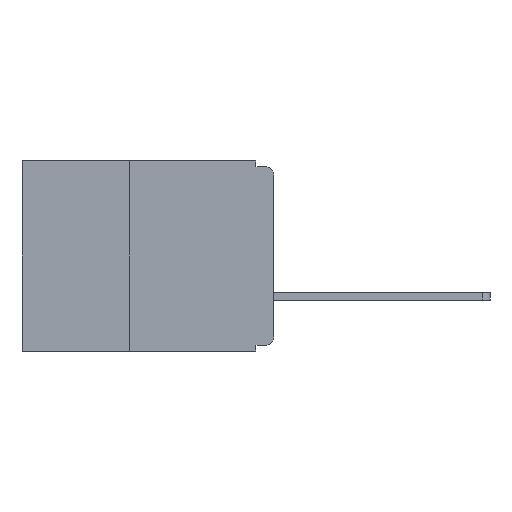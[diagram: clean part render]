
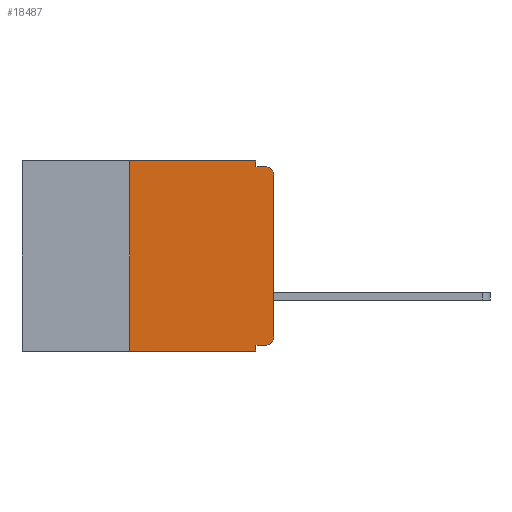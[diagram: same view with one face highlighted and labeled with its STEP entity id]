
A CAD part, left-side view. The second image highlights one B-rep face of the part: STEP entity #18487.
In plain terms, the highlighted planar face has unit normal (-1, 0, 0).
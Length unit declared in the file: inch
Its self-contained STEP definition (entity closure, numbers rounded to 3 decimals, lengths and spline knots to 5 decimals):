
#346 = LINE ( 'NONE', #22528, #4045 ) ;
#390 = ORIENTED_EDGE ( 'NONE', *, *, #810, .F. ) ;
#554 = CARTESIAN_POINT ( 'NONE',  ( 0., 0., -0.305 ) ) ;
#629 = ORIENTED_EDGE ( 'NONE', *, *, #4775, .T. ) ;
#810 = EDGE_CURVE ( 'NONE', #17981, #12182, #4354, .T. ) ;
#930 = DIRECTION ( 'NONE',  ( 0., 0., 1. ) ) ;
#1153 = PLANE ( 'NONE',  #10870 ) ;
#1577 = EDGE_CURVE ( 'NONE', #4454, #16784, #15068, .T. ) ;
#2307 = DIRECTION ( 'NONE',  ( -1., 0., 0. ) ) ;
#2333 = VECTOR ( 'NONE', #21687, 39.37008 ) ;
#2358 = DIRECTION ( 'NONE',  ( 0., 0., -1. ) ) ;
#2964 = DIRECTION ( 'NONE',  ( 0., 0., -1. ) ) ;
#4045 = VECTOR ( 'NONE', #930, 39.37008 ) ;
#4226 = LINE ( 'NONE', #22168, #21694 ) ;
#4227 = VECTOR ( 'NONE', #13757, 39.37008 ) ;
#4354 = LINE ( 'NONE', #13585, #18213 ) ;
#4454 = VERTEX_POINT ( 'NONE', #20474 ) ;
#4615 = VERTEX_POINT ( 'NONE', #11181 ) ;
#4775 = EDGE_CURVE ( 'NONE', #9815, #13558, #23043, .T. ) ;
#5423 = VERTEX_POINT ( 'NONE', #13109 ) ;
#5455 = VECTOR ( 'NONE', #10289, 39.37008 ) ;
#5767 = VECTOR ( 'NONE', #2358, 39.37008 ) ;
#5929 = EDGE_CURVE ( 'NONE', #4615, #17981, #7806, .T. ) ;
#6445 = FACE_OUTER_BOUND ( 'NONE', #19555, .T. ) ;
#7180 = CARTESIAN_POINT ( 'NONE',  ( 0., 0.015, -0.01 ) ) ;
#7247 = VECTOR ( 'NONE', #11694, 39.37008 ) ;
#7806 = LINE ( 'NONE', #11228, #7247 ) ;
#8665 = ORIENTED_EDGE ( 'NONE', *, *, #19623, .F. ) ;
#9010 = ORIENTED_EDGE ( 'NONE', *, *, #1577, .F. ) ;
#9106 = EDGE_CURVE ( 'NONE', #12182, #13558, #12610, .T. ) ;
#9701 = DIRECTION ( 'NONE',  ( 0., 0., 1. ) ) ;
#9815 = VERTEX_POINT ( 'NONE', #14717 ) ;
#10193 = LINE ( 'NONE', #17256, #4227 ) ;
#10289 = DIRECTION ( 'NONE',  ( 0., 1., 0. ) ) ;
#10312 = CARTESIAN_POINT ( 'NONE',  ( 0., 0., -0.32 ) ) ;
#10427 = EDGE_CURVE ( 'NONE', #4454, #21498, #19799, .T. ) ;
#10870 = AXIS2_PLACEMENT_3D ( 'NONE', #22728, #13884, #2964 ) ;
#11181 = CARTESIAN_POINT ( 'NONE',  ( 0., 0.25, 0. ) ) ;
#11228 = CARTESIAN_POINT ( 'NONE',  ( 0., 0.437, 0. ) ) ;
#11386 = EDGE_CURVE ( 'NONE', #15197, #5423, #10193, .T. ) ;
#11694 = DIRECTION ( 'NONE',  ( 0., -1., 0. ) ) ;
#11762 = ORIENTED_EDGE ( 'NONE', *, *, #17164, .T. ) ;
#12182 = VERTEX_POINT ( 'NONE', #23029 ) ;
#12610 = LINE ( 'NONE', #14586, #2333 ) ;
#12629 = CARTESIAN_POINT ( 'NONE',  ( 0., 0.031, -0.32 ) ) ;
#13109 = CARTESIAN_POINT ( 'NONE',  ( 0., 0.031, -0.33 ) ) ;
#13228 = CARTESIAN_POINT ( 'NONE',  ( 0., 0.015, -0.305 ) ) ;
#13427 = CARTESIAN_POINT ( 'NONE',  ( 0., 0.25, -0.33 ) ) ;
#13558 = VERTEX_POINT ( 'NONE', #7180 ) ;
#13585 = CARTESIAN_POINT ( 'NONE',  ( 0., 0.031, 0. ) ) ;
#13692 = DIRECTION ( 'NONE',  ( 0., 0., -1. ) ) ;
#13757 = DIRECTION ( 'NONE',  ( 0., -1., 0. ) ) ;
#13884 = DIRECTION ( 'NONE',  ( 1., 0., 0. ) ) ;
#14069 = AXIS2_PLACEMENT_3D ( 'NONE', #23110, #22999, #22953 ) ;
#14287 = CARTESIAN_POINT ( 'NONE',  ( 0., 0.031, 0. ) ) ;
#14586 = CARTESIAN_POINT ( 'NONE',  ( 0., 0., -0.01 ) ) ;
#14639 = EDGE_CURVE ( 'NONE', #16784, #5423, #15958, .T. ) ;
#14717 = CARTESIAN_POINT ( 'NONE',  ( 0., 0., -0.025 ) ) ;
#14906 = ORIENTED_EDGE ( 'NONE', *, *, #5929, .F. ) ;
#14991 = DIRECTION ( 'NONE',  ( 0., 0., -1. ) ) ;
#15068 = LINE ( 'NONE', #10312, #5455 ) ;
#15197 = VERTEX_POINT ( 'NONE', #13427 ) ;
#15499 = ORIENTED_EDGE ( 'NONE', *, *, #14639, .F. ) ;
#15781 = ORIENTED_EDGE ( 'NONE', *, *, #11386, .T. ) ;
#15958 = LINE ( 'NONE', #16769, #5767 ) ;
#16769 = CARTESIAN_POINT ( 'NONE',  ( 0., 0.031, -0.33 ) ) ;
#16784 = VERTEX_POINT ( 'NONE', #12629 ) ;
#17090 = ORIENTED_EDGE ( 'NONE', *, *, #9106, .F. ) ;
#17164 = EDGE_CURVE ( 'NONE', #21498, #9815, #4226, .T. ) ;
#17224 = ORIENTED_EDGE ( 'NONE', *, *, #10427, .T. ) ;
#17256 = CARTESIAN_POINT ( 'NONE',  ( 0., 0.437, -0.33 ) ) ;
#17981 = VERTEX_POINT ( 'NONE', #14287 ) ;
#18213 = VECTOR ( 'NONE', #13692, 39.37008 ) ;
#18487 = ADVANCED_FACE ( 'NONE', ( #6445 ), #1153, .F. ) ;
#19555 = EDGE_LOOP ( 'NONE', ( #11762, #629, #17090, #390, #14906, #8665, #15781, #15499, #9010, #17224 ) ) ;
#19623 = EDGE_CURVE ( 'NONE', #15197, #4615, #346, .T. ) ;
#19799 = CIRCLE ( 'NONE', #23018, 0.015 ) ;
#20474 = CARTESIAN_POINT ( 'NONE',  ( 0., 0.015, -0.32 ) ) ;
#21498 = VERTEX_POINT ( 'NONE', #554 ) ;
#21687 = DIRECTION ( 'NONE',  ( 0., -1., 0. ) ) ;
#21694 = VECTOR ( 'NONE', #9701, 39.37008 ) ;
#22168 = CARTESIAN_POINT ( 'NONE',  ( 0., 0., 0. ) ) ;
#22528 = CARTESIAN_POINT ( 'NONE',  ( 0., 0.25, -0.33 ) ) ;
#22728 = CARTESIAN_POINT ( 'NONE',  ( 0., 0.437, 0. ) ) ;
#22953 = DIRECTION ( 'NONE',  ( 0., 0., -1. ) ) ;
#22999 = DIRECTION ( 'NONE',  ( -1., 0., 0. ) ) ;
#23018 = AXIS2_PLACEMENT_3D ( 'NONE', #13228, #2307, #14991 ) ;
#23029 = CARTESIAN_POINT ( 'NONE',  ( 0., 0.031, -0.01 ) ) ;
#23043 = CIRCLE ( 'NONE', #14069, 0.015 ) ;
#23110 = CARTESIAN_POINT ( 'NONE',  ( 0., 0.015, -0.025 ) ) ;
